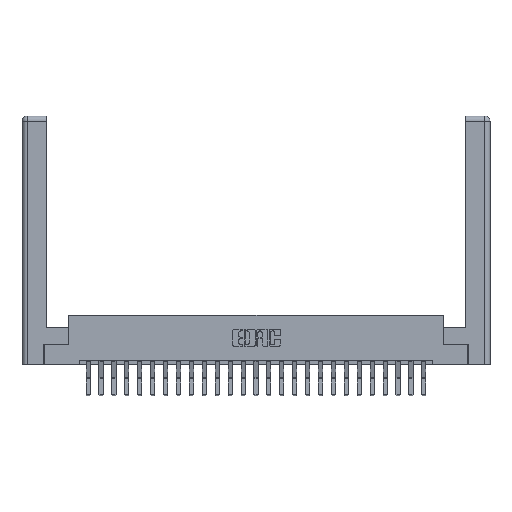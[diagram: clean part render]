
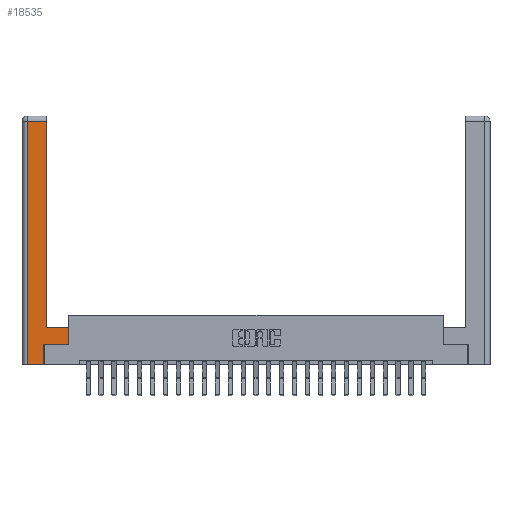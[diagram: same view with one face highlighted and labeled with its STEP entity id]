
A CAD part, top view. The second image highlights one B-rep face of the part: STEP entity #18535.
In plain terms, the highlighted planar face has unit normal (0, 0, 1).
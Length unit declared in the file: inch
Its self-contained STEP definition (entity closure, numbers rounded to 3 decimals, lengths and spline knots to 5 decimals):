
#113 = EDGE_CURVE ( 'NONE', #21837, #16218, #24502, .T. ) ;
#1329 = DIRECTION ( 'NONE',  ( -1., 0., 0. ) ) ;
#3038 = VERTEX_POINT ( 'NONE', #13423 ) ;
#3219 = VECTOR ( 'NONE', #9894, 39.37008 ) ;
#3509 = VERTEX_POINT ( 'NONE', #22578 ) ;
#3511 = LINE ( 'NONE', #15012, #25472 ) ;
#4189 = LINE ( 'NONE', #16868, #18704 ) ;
#4237 = VERTEX_POINT ( 'NONE', #24454 ) ;
#4520 = ORIENTED_EDGE ( 'NONE', *, *, #14961, .T. ) ;
#5410 = LINE ( 'NONE', #12502, #14341 ) ;
#6223 = ORIENTED_EDGE ( 'NONE', *, *, #22645, .T. ) ;
#7171 = CARTESIAN_POINT ( 'NONE',  ( 0.265, 0., 0. ) ) ;
#7553 = VECTOR ( 'NONE', #17447, 39.37008 ) ;
#7685 = CARTESIAN_POINT ( 'NONE',  ( 0.0615, 2.94, 0. ) ) ;
#8000 = VERTEX_POINT ( 'NONE', #18187 ) ;
#9894 = DIRECTION ( 'NONE',  ( -1., 0., 0. ) ) ;
#10101 = VECTOR ( 'NONE', #25354, 39.37008 ) ;
#10203 = ORIENTED_EDGE ( 'NONE', *, *, #19859, .T. ) ;
#10693 = ORIENTED_EDGE ( 'NONE', *, *, #113, .T. ) ;
#11052 = CARTESIAN_POINT ( 'NONE',  ( 0.565, 0.45, 0. ) ) ;
#12355 = AXIS2_PLACEMENT_3D ( 'NONE', #16900, #19136, #1329 ) ;
#12502 = CARTESIAN_POINT ( 'NONE',  ( 0.565, 0.45, 0. ) ) ;
#13423 = CARTESIAN_POINT ( 'NONE',  ( 0.265, 0., 0. ) ) ;
#13719 = EDGE_LOOP ( 'NONE', ( #19107, #6223, #4520, #25532, #10203, #19084, #18277, #10693 ) ) ;
#14020 = VERTEX_POINT ( 'NONE', #24505 ) ;
#14341 = VECTOR ( 'NONE', #18382, 39.37008 ) ;
#14410 = CARTESIAN_POINT ( 'NONE',  ( 0.295, 0.45, 0. ) ) ;
#14961 = EDGE_CURVE ( 'NONE', #3509, #14020, #3511, .T. ) ;
#15012 = CARTESIAN_POINT ( 'NONE',  ( 0.0615, 0., 0. ) ) ;
#15182 = CARTESIAN_POINT ( 'NONE',  ( 0.265, 0.245, 0. ) ) ;
#15863 = VERTEX_POINT ( 'NONE', #21769 ) ;
#16119 = VECTOR ( 'NONE', #19928, 39.37008 ) ;
#16218 = VERTEX_POINT ( 'NONE', #14410 ) ;
#16839 = VECTOR ( 'NONE', #25246, 39.37008 ) ;
#16868 = CARTESIAN_POINT ( 'NONE',  ( 0.295, 3., 0. ) ) ;
#16900 = CARTESIAN_POINT ( 'NONE',  ( 0., 0., 0. ) ) ;
#17447 = DIRECTION ( 'NONE',  ( 0., 1., 0. ) ) ;
#17770 = EDGE_CURVE ( 'NONE', #15863, #8000, #17865, .T. ) ;
#17865 = LINE ( 'NONE', #21432, #10101 ) ;
#18187 = CARTESIAN_POINT ( 'NONE',  ( 0.565, 0.245, 0. ) ) ;
#18198 = CARTESIAN_POINT ( 'NONE',  ( 0.295, 0.45, 0. ) ) ;
#18277 = ORIENTED_EDGE ( 'NONE', *, *, #22987, .T. ) ;
#18382 = DIRECTION ( 'NONE',  ( 0., 1., 0. ) ) ;
#18535 = ADVANCED_FACE ( 'NONE', ( #22785 ), #23131, .F. ) ;
#18704 = VECTOR ( 'NONE', #18844, 39.37008 ) ;
#18844 = DIRECTION ( 'NONE',  ( 0., 1., 0. ) ) ;
#19084 = ORIENTED_EDGE ( 'NONE', *, *, #17770, .T. ) ;
#19107 = ORIENTED_EDGE ( 'NONE', *, *, #19184, .T. ) ;
#19136 = DIRECTION ( 'NONE',  ( 0., 0., -1. ) ) ;
#19184 = EDGE_CURVE ( 'NONE', #16218, #4237, #4189, .T. ) ;
#19859 = EDGE_CURVE ( 'NONE', #3038, #15863, #24246, .T. ) ;
#19928 = DIRECTION ( 'NONE',  ( -1., 0., 0. ) ) ;
#20848 = LINE ( 'NONE', #7171, #16839 ) ;
#21432 = CARTESIAN_POINT ( 'NONE',  ( 0.565, 0.245, 0. ) ) ;
#21769 = CARTESIAN_POINT ( 'NONE',  ( 0.265, 0.245, 0. ) ) ;
#21837 = VERTEX_POINT ( 'NONE', #11052 ) ;
#22445 = EDGE_CURVE ( 'NONE', #14020, #3038, #20848, .T. ) ;
#22578 = CARTESIAN_POINT ( 'NONE',  ( 0.0615, 2.94, 0. ) ) ;
#22645 = EDGE_CURVE ( 'NONE', #4237, #3509, #24262, .T. ) ;
#22785 = FACE_OUTER_BOUND ( 'NONE', #13719, .T. ) ;
#22987 = EDGE_CURVE ( 'NONE', #8000, #21837, #5410, .T. ) ;
#23131 = PLANE ( 'NONE',  #12355 ) ;
#24246 = LINE ( 'NONE', #15182, #7553 ) ;
#24262 = LINE ( 'NONE', #7685, #3219 ) ;
#24454 = CARTESIAN_POINT ( 'NONE',  ( 0.295, 2.94, 0. ) ) ;
#24502 = LINE ( 'NONE', #18198, #16119 ) ;
#24505 = CARTESIAN_POINT ( 'NONE',  ( 0.0615, 0., 0. ) ) ;
#25246 = DIRECTION ( 'NONE',  ( 1., 0., 0. ) ) ;
#25331 = DIRECTION ( 'NONE',  ( 0., -1., 0. ) ) ;
#25354 = DIRECTION ( 'NONE',  ( 1., 0., 0. ) ) ;
#25472 = VECTOR ( 'NONE', #25331, 39.37008 ) ;
#25532 = ORIENTED_EDGE ( 'NONE', *, *, #22445, .T. ) ;
